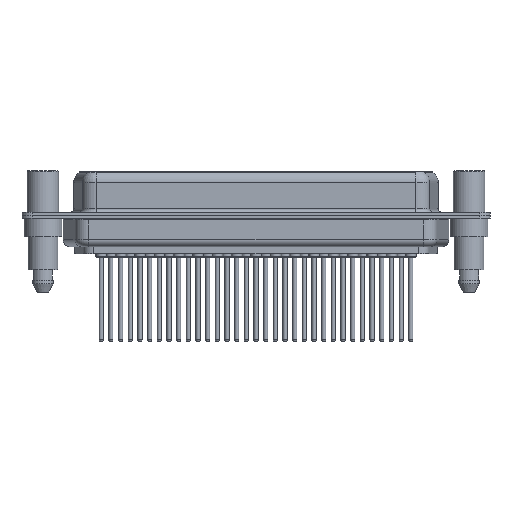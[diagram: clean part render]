
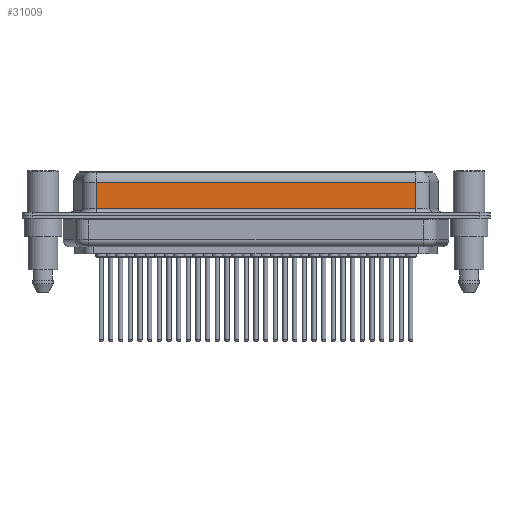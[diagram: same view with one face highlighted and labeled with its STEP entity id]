
A CAD part, front view. The second image highlights one B-rep face of the part: STEP entity #31009.
In plain terms, the highlighted planar face has unit normal (0, -1, 0).
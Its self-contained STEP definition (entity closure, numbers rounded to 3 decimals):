
#193 = VERTEX_POINT ( 'NONE', #14546 ) ;
#506 = LINE ( 'NONE', #26040, #3153 ) ;
#1014 = DIRECTION ( 'NONE',  ( 0., 1., 0. ) ) ;
#1033 = EDGE_CURVE ( 'NONE', #17753, #12713, #13300, .T. ) ;
#2412 = VERTEX_POINT ( 'NONE', #24279 ) ;
#3153 = VECTOR ( 'NONE', #17901, 1000. ) ;
#3384 = DIRECTION ( 'NONE',  ( -1., 0., 0. ) ) ;
#3403 = CARTESIAN_POINT ( 'NONE',  ( 53.383, -5.45, 6.4 ) ) ;
#3680 = CARTESIAN_POINT ( 'NONE',  ( 7.617, -5.45, 0.9 ) ) ;
#4129 = ORIENTED_EDGE ( 'NONE', *, *, #29839, .F. ) ;
#5463 = VECTOR ( 'NONE', #26071, 1000. ) ;
#8493 = FACE_OUTER_BOUND ( 'NONE', #23695, .T. ) ;
#12534 = AXIS2_PLACEMENT_3D ( 'NONE', #3403, #1014, #18560 ) ;
#12713 = VERTEX_POINT ( 'NONE', #3680 ) ;
#13300 = LINE ( 'NONE', #18521, #28784 ) ;
#14015 = PLANE ( 'NONE',  #12534 ) ;
#14546 = CARTESIAN_POINT ( 'NONE',  ( 53.383, -5.45, 4.65 ) ) ;
#15745 = LINE ( 'NONE', #31299, #5463 ) ;
#17753 = VERTEX_POINT ( 'NONE', #26661 ) ;
#17901 = DIRECTION ( 'NONE',  ( 1., 0., 0. ) ) ;
#18521 = CARTESIAN_POINT ( 'NONE',  ( 7.617, -5.45, 6.4 ) ) ;
#18560 = DIRECTION ( 'NONE',  ( 0., 0., 1. ) ) ;
#21269 = LINE ( 'NONE', #23977, #28673 ) ;
#22405 = ORIENTED_EDGE ( 'NONE', *, *, #33145, .T. ) ;
#23695 = EDGE_LOOP ( 'NONE', ( #4129, #22405, #29731, #26626 ) ) ;
#23977 = CARTESIAN_POINT ( 'NONE',  ( 53.383, -5.45, 4.65 ) ) ;
#24279 = CARTESIAN_POINT ( 'NONE',  ( 53.383, -5.45, 0.9 ) ) ;
#25759 = EDGE_CURVE ( 'NONE', #12713, #2412, #506, .T. ) ;
#26040 = CARTESIAN_POINT ( 'NONE',  ( 53.383, -5.45, 0.9 ) ) ;
#26071 = DIRECTION ( 'NONE',  ( 0., 0., -1. ) ) ;
#26329 = DIRECTION ( 'NONE',  ( 0., 0., -1. ) ) ;
#26626 = ORIENTED_EDGE ( 'NONE', *, *, #25759, .T. ) ;
#26661 = CARTESIAN_POINT ( 'NONE',  ( 7.617, -5.45, 4.65 ) ) ;
#28673 = VECTOR ( 'NONE', #3384, 1000. ) ;
#28784 = VECTOR ( 'NONE', #26329, 1000. ) ;
#29731 = ORIENTED_EDGE ( 'NONE', *, *, #1033, .T. ) ;
#29839 = EDGE_CURVE ( 'NONE', #193, #2412, #15745, .T. ) ;
#31009 = ADVANCED_FACE ( 'NONE', ( #8493 ), #14015, .F. ) ;
#31299 = CARTESIAN_POINT ( 'NONE',  ( 53.383, -5.45, 6.4 ) ) ;
#33145 = EDGE_CURVE ( 'NONE', #193, #17753, #21269, .T. ) ;
